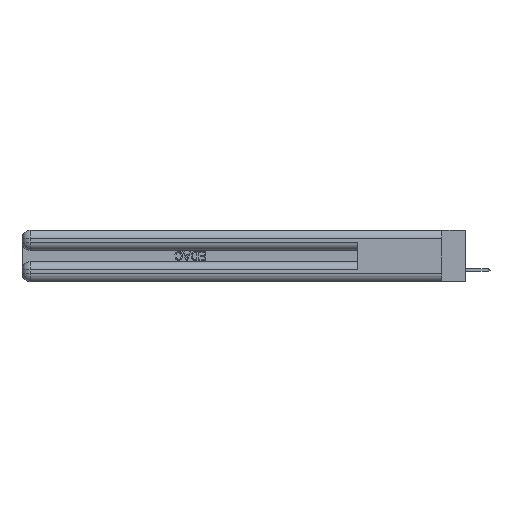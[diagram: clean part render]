
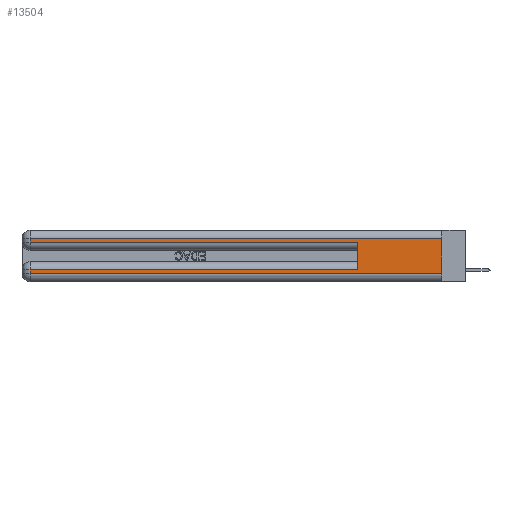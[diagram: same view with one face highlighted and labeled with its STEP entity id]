
A CAD part, left-side view. The second image highlights one B-rep face of the part: STEP entity #13504.
In plain terms, the highlighted planar face has unit normal (-1, 0, 0).
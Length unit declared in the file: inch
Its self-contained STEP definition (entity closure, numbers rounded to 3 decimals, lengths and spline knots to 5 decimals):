
#357 = LINE ( 'NONE', #12953, #17803 ) ;
#364 = CARTESIAN_POINT ( 'NONE',  ( 0., 0., 0.06 ) ) ;
#744 = LINE ( 'NONE', #16420, #16629 ) ;
#1114 = DIRECTION ( 'NONE',  ( 1., 0., 0. ) ) ;
#1451 = LINE ( 'NONE', #5588, #27387 ) ;
#1512 = ORIENTED_EDGE ( 'NONE', *, *, #9880, .T. ) ;
#2196 = VERTEX_POINT ( 'NONE', #28779 ) ;
#2505 = DIRECTION ( 'NONE',  ( 0., 1., 0. ) ) ;
#4866 = AXIS2_PLACEMENT_3D ( 'NONE', #24823, #1114, #11596 ) ;
#5511 = CARTESIAN_POINT ( 'NONE',  ( 0., 0.6, 0.085 ) ) ;
#5588 = CARTESIAN_POINT ( 'NONE',  ( 0., 0.6, 0.145 ) ) ;
#5679 = DIRECTION ( 'NONE',  ( 0., 0., -1. ) ) ;
#6543 = ORIENTED_EDGE ( 'NONE', *, *, #30142, .T. ) ;
#7213 = DIRECTION ( 'NONE',  ( 0., 0., -1. ) ) ;
#8398 = VERTEX_POINT ( 'NONE', #39248 ) ;
#8465 = ORIENTED_EDGE ( 'NONE', *, *, #29544, .T. ) ;
#9880 = EDGE_CURVE ( 'NONE', #28921, #11796, #357, .T. ) ;
#9902 = DIRECTION ( 'NONE',  ( 0., -1., 0. ) ) ;
#11219 = CARTESIAN_POINT ( 'NONE',  ( 0., 0.6, 0.285 ) ) ;
#11596 = DIRECTION ( 'NONE',  ( 0., 0., -1. ) ) ;
#11796 = VERTEX_POINT ( 'NONE', #364 ) ;
#11893 = DIRECTION ( 'NONE',  ( 0., 0., 1. ) ) ;
#12319 = CARTESIAN_POINT ( 'NONE',  ( 0., 0., 0.31 ) ) ;
#12876 = EDGE_CURVE ( 'NONE', #8398, #11796, #26701, .T. ) ;
#12953 = CARTESIAN_POINT ( 'NONE',  ( 0., 0., 0.06 ) ) ;
#13504 = ADVANCED_FACE ( 'NONE', ( #35061 ), #22022, .F. ) ;
#15093 = ORIENTED_EDGE ( 'NONE', *, *, #22762, .T. ) ;
#16420 = CARTESIAN_POINT ( 'NONE',  ( 0., 0., 0.285 ) ) ;
#16629 = VECTOR ( 'NONE', #9902, 39.37008 ) ;
#17624 = CARTESIAN_POINT ( 'NONE',  ( 0., 2.94, 0.285 ) ) ;
#17803 = VECTOR ( 'NONE', #19773, 39.37008 ) ;
#19704 = VERTEX_POINT ( 'NONE', #17624 ) ;
#19773 = DIRECTION ( 'NONE',  ( 0., -1., 0. ) ) ;
#20625 = VECTOR ( 'NONE', #34418, 39.37008 ) ;
#22022 = PLANE ( 'NONE',  #4866 ) ;
#22762 = EDGE_CURVE ( 'NONE', #33408, #34048, #31538, .T. ) ;
#24823 = CARTESIAN_POINT ( 'NONE',  ( 0., 0., 0.37 ) ) ;
#25115 = VECTOR ( 'NONE', #7213, 39.37008 ) ;
#25433 = LINE ( 'NONE', #40831, #20625 ) ;
#25758 = VECTOR ( 'NONE', #2505, 39.37008 ) ;
#25788 = CARTESIAN_POINT ( 'NONE',  ( 0., 0., 0.37 ) ) ;
#25971 = DIRECTION ( 'NONE',  ( 0., 1., 0. ) ) ;
#26169 = CARTESIAN_POINT ( 'NONE',  ( 0., 2.94, 0.06 ) ) ;
#26701 = LINE ( 'NONE', #25788, #38879 ) ;
#27387 = VECTOR ( 'NONE', #11893, 39.37008 ) ;
#27472 = CARTESIAN_POINT ( 'NONE',  ( 0., 2.94, 0.37 ) ) ;
#28779 = CARTESIAN_POINT ( 'NONE',  ( 0., 2.94, 0.31 ) ) ;
#28921 = VERTEX_POINT ( 'NONE', #26169 ) ;
#29544 = EDGE_CURVE ( 'NONE', #8398, #2196, #33145, .T. ) ;
#30142 = EDGE_CURVE ( 'NONE', #19704, #31030, #744, .T. ) ;
#30498 = VECTOR ( 'NONE', #25971, 39.37008 ) ;
#31030 = VERTEX_POINT ( 'NONE', #11219 ) ;
#31538 = LINE ( 'NONE', #32863, #25758 ) ;
#32772 = CARTESIAN_POINT ( 'NONE',  ( 0., 2.94, 0.085 ) ) ;
#32863 = CARTESIAN_POINT ( 'NONE',  ( 0., 0., 0.085 ) ) ;
#33145 = LINE ( 'NONE', #12319, #30498 ) ;
#33408 = VERTEX_POINT ( 'NONE', #5511 ) ;
#33917 = ORIENTED_EDGE ( 'NONE', *, *, #39164, .T. ) ;
#34048 = VERTEX_POINT ( 'NONE', #32772 ) ;
#34095 = LINE ( 'NONE', #27472, #25115 ) ;
#34418 = DIRECTION ( 'NONE',  ( 0., 0., -1. ) ) ;
#35061 = FACE_OUTER_BOUND ( 'NONE', #38092, .T. ) ;
#35510 = ORIENTED_EDGE ( 'NONE', *, *, #40525, .F. ) ;
#36704 = EDGE_CURVE ( 'NONE', #34048, #28921, #34095, .T. ) ;
#37287 = ORIENTED_EDGE ( 'NONE', *, *, #12876, .F. ) ;
#38031 = ORIENTED_EDGE ( 'NONE', *, *, #36704, .T. ) ;
#38092 = EDGE_LOOP ( 'NONE', ( #37287, #8465, #33917, #6543, #35510, #15093, #38031, #1512 ) ) ;
#38879 = VECTOR ( 'NONE', #5679, 39.37008 ) ;
#39164 = EDGE_CURVE ( 'NONE', #2196, #19704, #25433, .T. ) ;
#39248 = CARTESIAN_POINT ( 'NONE',  ( 0., 0., 0.31 ) ) ;
#40525 = EDGE_CURVE ( 'NONE', #33408, #31030, #1451, .T. ) ;
#40831 = CARTESIAN_POINT ( 'NONE',  ( 0., 2.94, 0.37 ) ) ;
